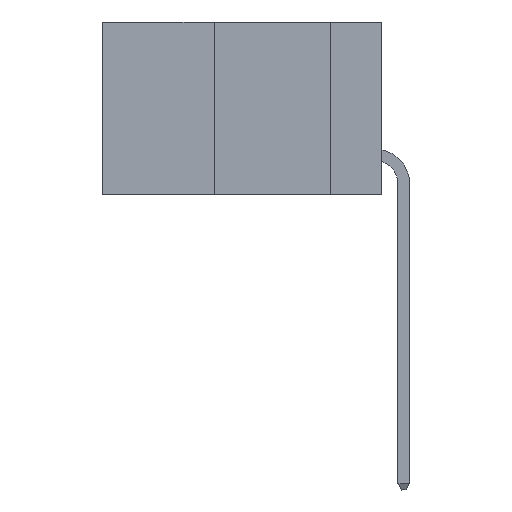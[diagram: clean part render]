
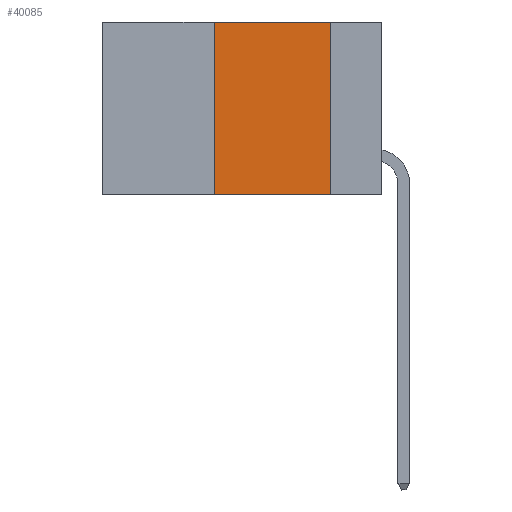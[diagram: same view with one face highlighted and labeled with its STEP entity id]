
A CAD part, left-side view. The second image highlights one B-rep face of the part: STEP entity #40085.
In plain terms, the highlighted planar face has unit normal (-1, 0, 0).
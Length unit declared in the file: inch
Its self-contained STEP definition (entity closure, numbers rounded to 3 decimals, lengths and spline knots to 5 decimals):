
#209 = LINE ( 'NONE', #2955, #42758 ) ;
#2955 = CARTESIAN_POINT ( 'NONE',  ( 0., 0.6, -0.37 ) ) ;
#5727 = LINE ( 'NONE', #31721, #15448 ) ;
#5763 = CARTESIAN_POINT ( 'NONE',  ( 0., 0.6, 0. ) ) ;
#11823 = CARTESIAN_POINT ( 'NONE',  ( 0., 0.11, -0.37 ) ) ;
#12812 = DIRECTION ( 'NONE',  ( 0., -1., 0. ) ) ;
#13071 = VERTEX_POINT ( 'NONE', #38669 ) ;
#13496 = EDGE_LOOP ( 'NONE', ( #45747, #30580, #31207, #26011 ) ) ;
#13524 = DIRECTION ( 'NONE',  ( 0., 0., -1. ) ) ;
#13673 = CARTESIAN_POINT ( 'NONE',  ( 0., 0.11, 0. ) ) ;
#14087 = DIRECTION ( 'NONE',  ( 0., -1., 0. ) ) ;
#15419 = EDGE_CURVE ( 'NONE', #17796, #22380, #5727, .T. ) ;
#15448 = VECTOR ( 'NONE', #12812, 39.37008 ) ;
#17796 = VERTEX_POINT ( 'NONE', #33776 ) ;
#20156 = EDGE_CURVE ( 'NONE', #13071, #34190, #209, .T. ) ;
#22380 = VERTEX_POINT ( 'NONE', #49489 ) ;
#25032 = VECTOR ( 'NONE', #43340, 39.37008 ) ;
#25234 = DIRECTION ( 'NONE',  ( 1., 0., 0. ) ) ;
#26011 = ORIENTED_EDGE ( 'NONE', *, *, #20156, .T. ) ;
#27476 = LINE ( 'NONE', #28160, #25032 ) ;
#28160 = CARTESIAN_POINT ( 'NONE',  ( 0., 0.36, 0. ) ) ;
#29129 = DIRECTION ( 'NONE',  ( 0., 0., -1. ) ) ;
#30580 = ORIENTED_EDGE ( 'NONE', *, *, #15419, .F. ) ;
#31207 = ORIENTED_EDGE ( 'NONE', *, *, #39347, .F. ) ;
#31304 = AXIS2_PLACEMENT_3D ( 'NONE', #5763, #25234, #13524 ) ;
#31721 = CARTESIAN_POINT ( 'NONE',  ( 0., 0.6, 0. ) ) ;
#33412 = PLANE ( 'NONE',  #31304 ) ;
#33776 = CARTESIAN_POINT ( 'NONE',  ( 0., 0.36, 0. ) ) ;
#34190 = VERTEX_POINT ( 'NONE', #11823 ) ;
#35498 = EDGE_CURVE ( 'NONE', #22380, #34190, #35767, .T. ) ;
#35767 = LINE ( 'NONE', #13673, #44927 ) ;
#38669 = CARTESIAN_POINT ( 'NONE',  ( 0., 0.36, -0.37 ) ) ;
#39347 = EDGE_CURVE ( 'NONE', #13071, #17796, #27476, .T. ) ;
#40085 = ADVANCED_FACE ( 'NONE', ( #40132 ), #33412, .F. ) ;
#40132 = FACE_OUTER_BOUND ( 'NONE', #13496, .T. ) ;
#42758 = VECTOR ( 'NONE', #14087, 39.37008 ) ;
#43340 = DIRECTION ( 'NONE',  ( 0., 0., 1. ) ) ;
#44927 = VECTOR ( 'NONE', #29129, 39.37008 ) ;
#45747 = ORIENTED_EDGE ( 'NONE', *, *, #35498, .F. ) ;
#49489 = CARTESIAN_POINT ( 'NONE',  ( 0., 0.11, 0. ) ) ;
